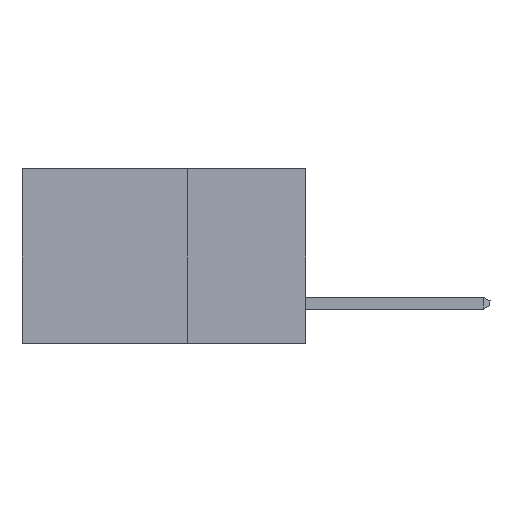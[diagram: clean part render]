
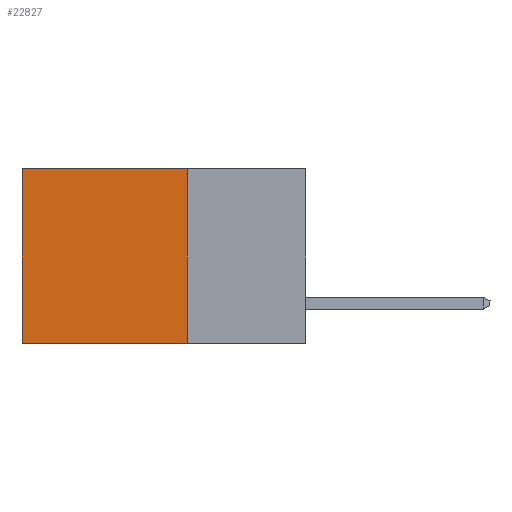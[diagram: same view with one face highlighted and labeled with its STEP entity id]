
A CAD part, left-side view. The second image highlights one B-rep face of the part: STEP entity #22827.
In plain terms, the highlighted planar face has unit normal (-1, 0, 0).
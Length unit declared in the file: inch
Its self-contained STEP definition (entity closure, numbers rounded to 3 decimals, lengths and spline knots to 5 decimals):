
#515 = VERTEX_POINT ( 'NONE', #19717 ) ;
#1049 = VECTOR ( 'NONE', #18962, 39.37008 ) ;
#1411 = LINE ( 'NONE', #11318, #1049 ) ;
#1538 = LINE ( 'NONE', #6903, #3116 ) ;
#2160 = ORIENTED_EDGE ( 'NONE', *, *, #4575, .T. ) ;
#2772 = CARTESIAN_POINT ( 'NONE',  ( 0.2615, 0.6, 0. ) ) ;
#3116 = VECTOR ( 'NONE', #20778, 39.37008 ) ;
#3948 = EDGE_CURVE ( 'NONE', #515, #24005, #5764, .T. ) ;
#4212 = DIRECTION ( 'NONE',  ( 1., 0., 0. ) ) ;
#4575 = EDGE_CURVE ( 'NONE', #515, #19576, #1538, .T. ) ;
#4582 = EDGE_CURVE ( 'NONE', #24005, #18994, #1411, .T. ) ;
#5764 = LINE ( 'NONE', #9554, #22291 ) ;
#6450 = DIRECTION ( 'NONE',  ( 0., 0., -1. ) ) ;
#6903 = CARTESIAN_POINT ( 'NONE',  ( 0.2615, 0.25, 0. ) ) ;
#7551 = CARTESIAN_POINT ( 'NONE',  ( 0.2615, 0.6, -0.37 ) ) ;
#9554 = CARTESIAN_POINT ( 'NONE',  ( 0.2615, 0.25, -0.37 ) ) ;
#10228 = CARTESIAN_POINT ( 'NONE',  ( 0.2615, 0.25, -0.37 ) ) ;
#11083 = LINE ( 'NONE', #7551, #23652 ) ;
#11318 = CARTESIAN_POINT ( 'NONE',  ( 0.2615, 0.25, -0.37 ) ) ;
#14612 = FACE_OUTER_BOUND ( 'NONE', #19127, .T. ) ;
#14932 = AXIS2_PLACEMENT_3D ( 'NONE', #10228, #4212, #6450 ) ;
#15012 = ORIENTED_EDGE ( 'NONE', *, *, #3948, .F. ) ;
#17455 = DIRECTION ( 'NONE',  ( 0., 0., -1. ) ) ;
#18017 = CARTESIAN_POINT ( 'NONE',  ( 0.2615, 0.6, -0.37 ) ) ;
#18962 = DIRECTION ( 'NONE',  ( 0., 1., 0. ) ) ;
#18994 = VERTEX_POINT ( 'NONE', #18017 ) ;
#19127 = EDGE_LOOP ( 'NONE', ( #21872, #25202, #15012, #2160 ) ) ;
#19576 = VERTEX_POINT ( 'NONE', #2772 ) ;
#19717 = CARTESIAN_POINT ( 'NONE',  ( 0.2615, 0.25, 0. ) ) ;
#20778 = DIRECTION ( 'NONE',  ( 0., 1., 0. ) ) ;
#21872 = ORIENTED_EDGE ( 'NONE', *, *, #22166, .T. ) ;
#22166 = EDGE_CURVE ( 'NONE', #19576, #18994, #11083, .T. ) ;
#22291 = VECTOR ( 'NONE', #17455, 39.37008 ) ;
#22565 = PLANE ( 'NONE',  #14932 ) ;
#22827 = ADVANCED_FACE ( 'NONE', ( #14612 ), #22565, .F. ) ;
#22876 = CARTESIAN_POINT ( 'NONE',  ( 0.2615, 0.25, -0.37 ) ) ;
#23031 = DIRECTION ( 'NONE',  ( 0., 0., -1. ) ) ;
#23652 = VECTOR ( 'NONE', #23031, 39.37008 ) ;
#24005 = VERTEX_POINT ( 'NONE', #22876 ) ;
#25202 = ORIENTED_EDGE ( 'NONE', *, *, #4582, .F. ) ;
